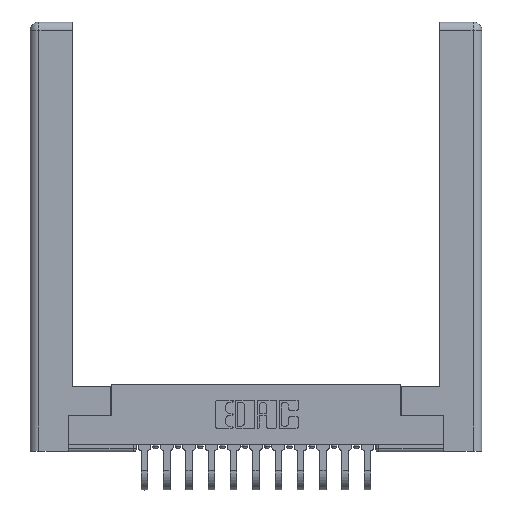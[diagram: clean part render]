
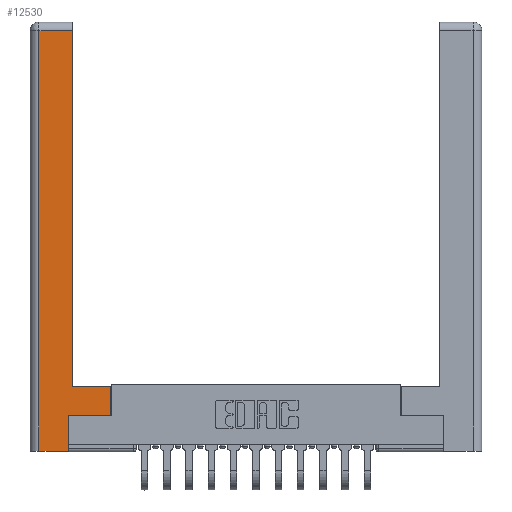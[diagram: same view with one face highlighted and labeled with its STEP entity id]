
A CAD part, top view. The second image highlights one B-rep face of the part: STEP entity #12530.
In plain terms, the highlighted planar face has unit normal (0, 0, 1).
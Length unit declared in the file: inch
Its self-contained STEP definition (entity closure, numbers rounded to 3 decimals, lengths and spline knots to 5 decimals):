
#174 = VERTEX_POINT ( 'NONE', #11023 ) ;
#1057 = EDGE_CURVE ( 'NONE', #174, #14298, #3599, .T. ) ;
#1096 = VERTEX_POINT ( 'NONE', #15662 ) ;
#1171 = LINE ( 'NONE', #13615, #2764 ) ;
#1305 = EDGE_CURVE ( 'NONE', #14298, #1096, #15417, .T. ) ;
#1441 = CARTESIAN_POINT ( 'NONE',  ( 0.565, 0.45, 0. ) ) ;
#1573 = LINE ( 'NONE', #5370, #9545 ) ;
#1657 = EDGE_CURVE ( 'NONE', #13617, #10660, #1171, .T. ) ;
#2076 = CARTESIAN_POINT ( 'NONE',  ( 0.0615, 0., 0. ) ) ;
#2661 = EDGE_LOOP ( 'NONE', ( #6865, #9733, #6957, #9154, #6564, #13397, #2814, #13769 ) ) ;
#2739 = VECTOR ( 'NONE', #10966, 39.37008 ) ;
#2764 = VECTOR ( 'NONE', #11017, 39.37008 ) ;
#2814 = ORIENTED_EDGE ( 'NONE', *, *, #1657, .T. ) ;
#3266 = DIRECTION ( 'NONE',  ( -1., 0., 0. ) ) ;
#3551 = CARTESIAN_POINT ( 'NONE',  ( 0.265, 0., 0. ) ) ;
#3577 = VECTOR ( 'NONE', #8053, 39.37008 ) ;
#3599 = LINE ( 'NONE', #8543, #2739 ) ;
#3998 = EDGE_CURVE ( 'NONE', #8215, #12106, #6598, .T. ) ;
#4096 = EDGE_CURVE ( 'NONE', #15803, #8215, #1573, .T. ) ;
#4246 = DIRECTION ( 'NONE',  ( -1., 0., 0. ) ) ;
#4328 = CARTESIAN_POINT ( 'NONE',  ( 0.0615, 0., 0. ) ) ;
#4566 = CARTESIAN_POINT ( 'NONE',  ( 0., 0., 0. ) ) ;
#5370 = CARTESIAN_POINT ( 'NONE',  ( 0.265, 0., 0. ) ) ;
#5434 = VECTOR ( 'NONE', #12978, 39.37008 ) ;
#6523 = CARTESIAN_POINT ( 'NONE',  ( 0.295, 2.94, 0. ) ) ;
#6564 = ORIENTED_EDGE ( 'NONE', *, *, #3998, .T. ) ;
#6598 = LINE ( 'NONE', #11532, #10849 ) ;
#6865 = ORIENTED_EDGE ( 'NONE', *, *, #1057, .T. ) ;
#6957 = ORIENTED_EDGE ( 'NONE', *, *, #12532, .T. ) ;
#7866 = CARTESIAN_POINT ( 'NONE',  ( 0.565, 0.245, 0. ) ) ;
#7948 = DIRECTION ( 'NONE',  ( 1., 0., 0. ) ) ;
#8053 = DIRECTION ( 'NONE',  ( 0., -1., 0. ) ) ;
#8204 = LINE ( 'NONE', #4328, #3577 ) ;
#8215 = VERTEX_POINT ( 'NONE', #3551 ) ;
#8543 = CARTESIAN_POINT ( 'NONE',  ( 0.295, 3., 0. ) ) ;
#8672 = CARTESIAN_POINT ( 'NONE',  ( 0.265, 0.245, 0. ) ) ;
#8959 = VECTOR ( 'NONE', #4246, 39.37008 ) ;
#9154 = ORIENTED_EDGE ( 'NONE', *, *, #4096, .T. ) ;
#9173 = DIRECTION ( 'NONE',  ( 0., 1., 0. ) ) ;
#9545 = VECTOR ( 'NONE', #7948, 39.37008 ) ;
#9733 = ORIENTED_EDGE ( 'NONE', *, *, #1305, .T. ) ;
#9858 = PLANE ( 'NONE',  #10549 ) ;
#10260 = DIRECTION ( 'NONE',  ( 0., 0., -1. ) ) ;
#10393 = LINE ( 'NONE', #15345, #8959 ) ;
#10549 = AXIS2_PLACEMENT_3D ( 'NONE', #4566, #10260, #3266 ) ;
#10660 = VERTEX_POINT ( 'NONE', #1441 ) ;
#10849 = VECTOR ( 'NONE', #9173, 39.37008 ) ;
#10966 = DIRECTION ( 'NONE',  ( 0., 1., 0. ) ) ;
#11017 = DIRECTION ( 'NONE',  ( 0., 1., 0. ) ) ;
#11023 = CARTESIAN_POINT ( 'NONE',  ( 0.295, 0.45, 0. ) ) ;
#11532 = CARTESIAN_POINT ( 'NONE',  ( 0.265, 0.245, 0. ) ) ;
#12106 = VERTEX_POINT ( 'NONE', #8672 ) ;
#12530 = ADVANCED_FACE ( 'NONE', ( #16006 ), #9858, .F. ) ;
#12532 = EDGE_CURVE ( 'NONE', #1096, #15803, #8204, .T. ) ;
#12978 = DIRECTION ( 'NONE',  ( -1., 0., 0. ) ) ;
#13333 = DIRECTION ( 'NONE',  ( 1., 0., 0. ) ) ;
#13397 = ORIENTED_EDGE ( 'NONE', *, *, #15390, .T. ) ;
#13615 = CARTESIAN_POINT ( 'NONE',  ( 0.565, 0.45, 0. ) ) ;
#13617 = VERTEX_POINT ( 'NONE', #7866 ) ;
#13769 = ORIENTED_EDGE ( 'NONE', *, *, #14315, .T. ) ;
#14298 = VERTEX_POINT ( 'NONE', #6523 ) ;
#14315 = EDGE_CURVE ( 'NONE', #10660, #174, #10393, .T. ) ;
#14476 = LINE ( 'NONE', #15999, #15713 ) ;
#15345 = CARTESIAN_POINT ( 'NONE',  ( 0.295, 0.45, 0. ) ) ;
#15390 = EDGE_CURVE ( 'NONE', #12106, #13617, #14476, .T. ) ;
#15417 = LINE ( 'NONE', #15494, #5434 ) ;
#15494 = CARTESIAN_POINT ( 'NONE',  ( 0.0615, 2.94, 0. ) ) ;
#15662 = CARTESIAN_POINT ( 'NONE',  ( 0.0615, 2.94, 0. ) ) ;
#15713 = VECTOR ( 'NONE', #13333, 39.37008 ) ;
#15803 = VERTEX_POINT ( 'NONE', #2076 ) ;
#15999 = CARTESIAN_POINT ( 'NONE',  ( 0.565, 0.245, 0. ) ) ;
#16006 = FACE_OUTER_BOUND ( 'NONE', #2661, .T. ) ;
